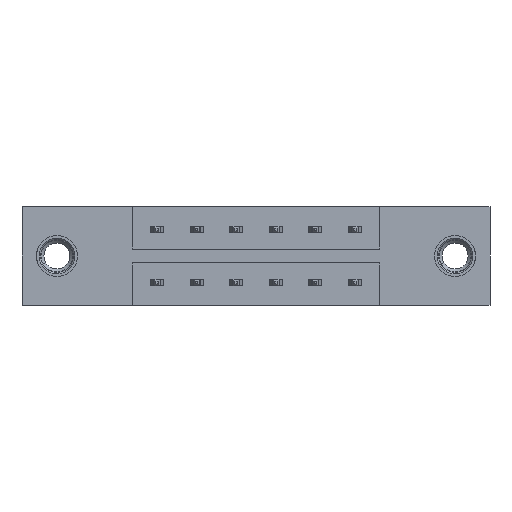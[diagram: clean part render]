
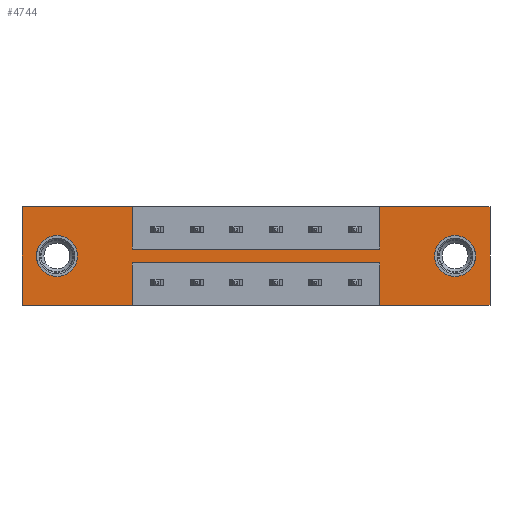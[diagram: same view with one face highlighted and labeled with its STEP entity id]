
A CAD part, front view. The second image highlights one B-rep face of the part: STEP entity #4744.
In plain terms, the highlighted planar face has unit normal (0, -1, 0).
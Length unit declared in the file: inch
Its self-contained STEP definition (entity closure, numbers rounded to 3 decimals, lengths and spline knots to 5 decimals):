
#21 = VERTEX_POINT ( 'NONE', #5267 ) ;
#29 = LINE ( 'NONE', #6449, #4502 ) ;
#39 = VECTOR ( 'NONE', #5833, 39.37008 ) ;
#66 = CIRCLE ( 'NONE', #4887, 0.078 ) ;
#599 = DIRECTION ( 'NONE',  ( 0., 0., 1. ) ) ;
#721 = DIRECTION ( 'NONE',  ( 1., 0., 0. ) ) ;
#730 = CARTESIAN_POINT ( 'NONE',  ( 0.4175, 0., -0.161 ) ) ;
#858 = LINE ( 'NONE', #4138, #7326 ) ;
#911 = VECTOR ( 'NONE', #8857, 39.37008 ) ;
#947 = EDGE_CURVE ( 'NONE', #2149, #3343, #6400, .T. ) ;
#987 = CARTESIAN_POINT ( 'NONE',  ( 1.6425, 0., -0.2655 ) ) ;
#1046 = LINE ( 'NONE', #5265, #9151 ) ;
#1205 = PLANE ( 'NONE',  #8171 ) ;
#1222 = EDGE_CURVE ( 'NONE', #7889, #9574, #858, .T. ) ;
#1295 = ORIENTED_EDGE ( 'NONE', *, *, #7106, .F. ) ;
#1321 = DIRECTION ( 'NONE',  ( -1., 0., 0. ) ) ;
#1481 = FACE_BOUND ( 'NONE', #3884, .T. ) ;
#1514 = DIRECTION ( 'NONE',  ( 0., 0., 1. ) ) ;
#1573 = EDGE_CURVE ( 'NONE', #5201, #21, #2159, .T. ) ;
#1868 = CIRCLE ( 'NONE', #4934, 0.078 ) ;
#1912 = VERTEX_POINT ( 'NONE', #3106 ) ;
#1964 = DIRECTION ( 'NONE',  ( 0., 0., -1. ) ) ;
#2024 = CARTESIAN_POINT ( 'NONE',  ( 0., 0., -0.375 ) ) ;
#2051 = LINE ( 'NONE', #8190, #39 ) ;
#2149 = VERTEX_POINT ( 'NONE', #4922 ) ;
#2159 = LINE ( 'NONE', #5278, #9670 ) ;
#2198 = DIRECTION ( 'NONE',  ( 0., 1., 0. ) ) ;
#2200 = CARTESIAN_POINT ( 'NONE',  ( 1.3575, 0., 0. ) ) ;
#2270 = DIRECTION ( 'NONE',  ( 0., 0., 1. ) ) ;
#2384 = DIRECTION ( 'NONE',  ( 0., 1., 0. ) ) ;
#2842 = CARTESIAN_POINT ( 'NONE',  ( 0., 0., -0.375 ) ) ;
#2861 = VERTEX_POINT ( 'NONE', #8807 ) ;
#2869 = DIRECTION ( 'NONE',  ( 0., 0., -1. ) ) ;
#2917 = LINE ( 'NONE', #4306, #911 ) ;
#2998 = VECTOR ( 'NONE', #8096, 39.37008 ) ;
#3001 = DIRECTION ( 'NONE',  ( 0., 1., 0. ) ) ;
#3106 = CARTESIAN_POINT ( 'NONE',  ( 0., 0., 0. ) ) ;
#3160 = CARTESIAN_POINT ( 'NONE',  ( 0.4175, 0., -0.161 ) ) ;
#3192 = LINE ( 'NONE', #3759, #7579 ) ;
#3202 = ORIENTED_EDGE ( 'NONE', *, *, #1222, .F. ) ;
#3269 = FACE_OUTER_BOUND ( 'NONE', #4279, .T. ) ;
#3343 = VERTEX_POINT ( 'NONE', #987 ) ;
#3371 = VERTEX_POINT ( 'NONE', #2200 ) ;
#3373 = EDGE_CURVE ( 'NONE', #8458, #1912, #3192, .T. ) ;
#3630 = CARTESIAN_POINT ( 'NONE',  ( 0.4175, 0., 0. ) ) ;
#3759 = CARTESIAN_POINT ( 'NONE',  ( 0., 0., 0. ) ) ;
#3774 = DIRECTION ( 'NONE',  ( 0., 0., 1. ) ) ;
#3884 = EDGE_LOOP ( 'NONE', ( #7760, #7211 ) ) ;
#4016 = ORIENTED_EDGE ( 'NONE', *, *, #5853, .F. ) ;
#4043 = VERTEX_POINT ( 'NONE', #6964 ) ;
#4059 = ORIENTED_EDGE ( 'NONE', *, *, #4386, .F. ) ;
#4138 = CARTESIAN_POINT ( 'NONE',  ( 0.4175, 0., -0.214 ) ) ;
#4279 = EDGE_LOOP ( 'NONE', ( #4059, #7510, #9110, #9350, #4016, #7670, #1295, #6779, #6697, #8886, #3202, #5087 ) ) ;
#4306 = CARTESIAN_POINT ( 'NONE',  ( 0., 0., 0. ) ) ;
#4353 = VERTEX_POINT ( 'NONE', #5100 ) ;
#4386 = EDGE_CURVE ( 'NONE', #4353, #7186, #8494, .T. ) ;
#4400 = EDGE_CURVE ( 'NONE', #3371, #5201, #1046, .T. ) ;
#4502 = VECTOR ( 'NONE', #1321, 39.37008 ) ;
#4710 = ORIENTED_EDGE ( 'NONE', *, *, #8721, .T. ) ;
#4744 = ADVANCED_FACE ( 'NONE', ( #1481, #7238, #3269 ), #1205, .T. ) ;
#4887 = AXIS2_PLACEMENT_3D ( 'NONE', #7446, #3001, #5154 ) ;
#4922 = CARTESIAN_POINT ( 'NONE',  ( 1.6425, 0., -0.1095 ) ) ;
#4934 = AXIS2_PLACEMENT_3D ( 'NONE', #6011, #2384, #3774 ) ;
#5087 = ORIENTED_EDGE ( 'NONE', *, *, #5726, .F. ) ;
#5100 = CARTESIAN_POINT ( 'NONE',  ( 1.3575, 0., -0.375 ) ) ;
#5154 = DIRECTION ( 'NONE',  ( 0., 0., -1. ) ) ;
#5201 = VERTEX_POINT ( 'NONE', #5397 ) ;
#5265 = CARTESIAN_POINT ( 'NONE',  ( 0., 0., 0. ) ) ;
#5267 = CARTESIAN_POINT ( 'NONE',  ( 1.775, 0., -0.375 ) ) ;
#5278 = CARTESIAN_POINT ( 'NONE',  ( 1.775, 0., 0. ) ) ;
#5301 = EDGE_CURVE ( 'NONE', #9574, #8458, #2051, .T. ) ;
#5393 = CARTESIAN_POINT ( 'NONE',  ( 0.4175, 0., -0.214 ) ) ;
#5397 = CARTESIAN_POINT ( 'NONE',  ( 1.775, 0., 0. ) ) ;
#5445 = DIRECTION ( 'NONE',  ( 0., 1., 0. ) ) ;
#5509 = CARTESIAN_POINT ( 'NONE',  ( 0.1325, 0., -0.1875 ) ) ;
#5583 = DIRECTION ( 'NONE',  ( 0., 0., -1. ) ) ;
#5603 = EDGE_CURVE ( 'NONE', #21, #4353, #29, .T. ) ;
#5634 = VECTOR ( 'NONE', #7554, 39.37008 ) ;
#5726 = EDGE_CURVE ( 'NONE', #7186, #7889, #8970, .T. ) ;
#5833 = DIRECTION ( 'NONE',  ( -1., 0., 0. ) ) ;
#5853 = EDGE_CURVE ( 'NONE', #4043, #3371, #8253, .T. ) ;
#5867 = VERTEX_POINT ( 'NONE', #6099 ) ;
#6011 = CARTESIAN_POINT ( 'NONE',  ( 0.1325, 0., -0.1875 ) ) ;
#6075 = DIRECTION ( 'NONE',  ( 0., 0., -1. ) ) ;
#6099 = CARTESIAN_POINT ( 'NONE',  ( 0.1325, 0., -0.2655 ) ) ;
#6253 = DIRECTION ( 'NONE',  ( 0., 0., 1. ) ) ;
#6346 = VERTEX_POINT ( 'NONE', #3630 ) ;
#6400 = CIRCLE ( 'NONE', #9134, 0.078 ) ;
#6404 = CARTESIAN_POINT ( 'NONE',  ( 0.4175, 0., -0.375 ) ) ;
#6449 = CARTESIAN_POINT ( 'NONE',  ( 0., 0., -0.375 ) ) ;
#6452 = AXIS2_PLACEMENT_3D ( 'NONE', #5509, #5445, #6253 ) ;
#6461 = DIRECTION ( 'NONE',  ( 0., -1., 0. ) ) ;
#6623 = CARTESIAN_POINT ( 'NONE',  ( 1.6425, 0., -0.1875 ) ) ;
#6697 = ORIENTED_EDGE ( 'NONE', *, *, #3373, .F. ) ;
#6779 = ORIENTED_EDGE ( 'NONE', *, *, #9120, .F. ) ;
#6780 = EDGE_LOOP ( 'NONE', ( #9651, #4710 ) ) ;
#6854 = CARTESIAN_POINT ( 'NONE',  ( 1.3575, 0., -0.161 ) ) ;
#6964 = CARTESIAN_POINT ( 'NONE',  ( 1.3575, 0., -0.161 ) ) ;
#7106 = EDGE_CURVE ( 'NONE', #6346, #8366, #7892, .T. ) ;
#7112 = VECTOR ( 'NONE', #2270, 39.37008 ) ;
#7186 = VERTEX_POINT ( 'NONE', #7522 ) ;
#7211 = ORIENTED_EDGE ( 'NONE', *, *, #9253, .T. ) ;
#7238 = FACE_BOUND ( 'NONE', #6780, .T. ) ;
#7315 = DIRECTION ( 'NONE',  ( 0., 0., -1. ) ) ;
#7326 = VECTOR ( 'NONE', #5583, 39.37008 ) ;
#7446 = CARTESIAN_POINT ( 'NONE',  ( 1.6425, 0., -0.1875 ) ) ;
#7510 = ORIENTED_EDGE ( 'NONE', *, *, #5603, .F. ) ;
#7522 = CARTESIAN_POINT ( 'NONE',  ( 1.3575, 0., -0.214 ) ) ;
#7554 = DIRECTION ( 'NONE',  ( 1., 0., 0. ) ) ;
#7579 = VECTOR ( 'NONE', #1514, 39.37008 ) ;
#7670 = ORIENTED_EDGE ( 'NONE', *, *, #8609, .F. ) ;
#7760 = ORIENTED_EDGE ( 'NONE', *, *, #947, .T. ) ;
#7889 = VERTEX_POINT ( 'NONE', #5393 ) ;
#7892 = LINE ( 'NONE', #730, #9317 ) ;
#8096 = DIRECTION ( 'NONE',  ( -1., 0., 0. ) ) ;
#8171 = AXIS2_PLACEMENT_3D ( 'NONE', #2024, #6461, #1964 ) ;
#8190 = CARTESIAN_POINT ( 'NONE',  ( 0., 0., -0.375 ) ) ;
#8192 = LINE ( 'NONE', #9072, #5634 ) ;
#8235 = CARTESIAN_POINT ( 'NONE',  ( 0.4175, 0., -0.214 ) ) ;
#8253 = LINE ( 'NONE', #6854, #7112 ) ;
#8366 = VERTEX_POINT ( 'NONE', #3160 ) ;
#8458 = VERTEX_POINT ( 'NONE', #2842 ) ;
#8494 = LINE ( 'NONE', #9603, #9212 ) ;
#8609 = EDGE_CURVE ( 'NONE', #8366, #4043, #8192, .T. ) ;
#8662 = EDGE_CURVE ( 'NONE', #2861, #5867, #1868, .T. ) ;
#8721 = EDGE_CURVE ( 'NONE', #5867, #2861, #9620, .T. ) ;
#8807 = CARTESIAN_POINT ( 'NONE',  ( 0.1325, 0., -0.1095 ) ) ;
#8857 = DIRECTION ( 'NONE',  ( 1., 0., 0. ) ) ;
#8886 = ORIENTED_EDGE ( 'NONE', *, *, #5301, .F. ) ;
#8970 = LINE ( 'NONE', #8235, #2998 ) ;
#9072 = CARTESIAN_POINT ( 'NONE',  ( 0.4175, 0., -0.161 ) ) ;
#9110 = ORIENTED_EDGE ( 'NONE', *, *, #1573, .F. ) ;
#9120 = EDGE_CURVE ( 'NONE', #1912, #6346, #2917, .T. ) ;
#9134 = AXIS2_PLACEMENT_3D ( 'NONE', #6623, #2198, #7315 ) ;
#9151 = VECTOR ( 'NONE', #721, 39.37008 ) ;
#9212 = VECTOR ( 'NONE', #599, 39.37008 ) ;
#9253 = EDGE_CURVE ( 'NONE', #3343, #2149, #66, .T. ) ;
#9317 = VECTOR ( 'NONE', #6075, 39.37008 ) ;
#9350 = ORIENTED_EDGE ( 'NONE', *, *, #4400, .F. ) ;
#9574 = VERTEX_POINT ( 'NONE', #6404 ) ;
#9603 = CARTESIAN_POINT ( 'NONE',  ( 1.3575, 0., -0.214 ) ) ;
#9620 = CIRCLE ( 'NONE', #6452, 0.078 ) ;
#9651 = ORIENTED_EDGE ( 'NONE', *, *, #8662, .T. ) ;
#9670 = VECTOR ( 'NONE', #2869, 39.37008 ) ;
